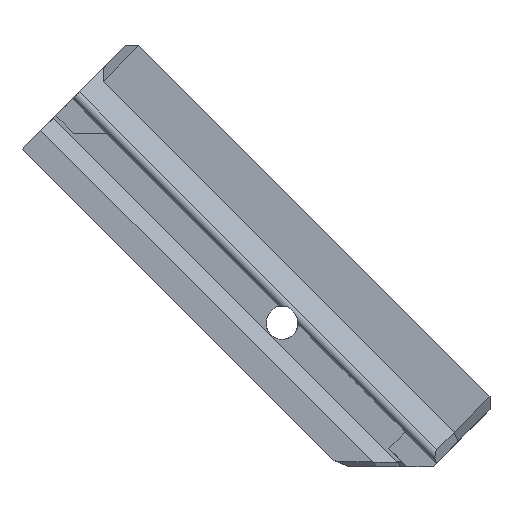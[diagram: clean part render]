
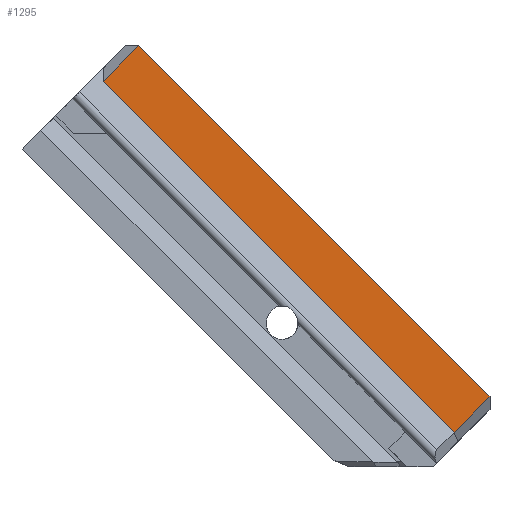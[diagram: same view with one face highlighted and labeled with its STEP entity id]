
A CAD part, left-side view. The second image highlights one B-rep face of the part: STEP entity #1295.
In plain terms, the highlighted planar face has unit normal (-1, 0, 0).
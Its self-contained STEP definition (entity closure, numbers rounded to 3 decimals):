
#69=FACE_OUTER_BOUND('',#141,.T.);
#141=EDGE_LOOP('',(#921,#922,#923,#924));
#245=LINE('',#1895,#410);
#255=LINE('',#1916,#420);
#259=LINE('',#1924,#424);
#260=LINE('',#1925,#425);
#410=VECTOR('',#1521,10.);
#420=VECTOR('',#1543,10.);
#424=VECTOR('',#1549,10.);
#425=VECTOR('',#1550,10.);
#567=VERTEX_POINT('',#1884);
#568=VERTEX_POINT('',#1889);
#574=VERTEX_POINT('',#1915);
#577=VERTEX_POINT('',#1923);
#695=EDGE_CURVE('',#567,#568,#245,.T.);
#705=EDGE_CURVE('',#568,#574,#255,.T.);
#709=EDGE_CURVE('',#567,#577,#259,.T.);
#710=EDGE_CURVE('',#574,#577,#260,.T.);
#921=ORIENTED_EDGE('',*,*,#695,.F.);
#922=ORIENTED_EDGE('',*,*,#709,.T.);
#923=ORIENTED_EDGE('',*,*,#710,.F.);
#924=ORIENTED_EDGE('',*,*,#705,.F.);
#1231=PLANE('',#1383);
#1295=ADVANCED_FACE('',(#69),#1231,.F.);
#1383=AXIS2_PLACEMENT_3D('',#1922,#1547,#1548);
#1521=DIRECTION('',(0.,0.707,-0.707));
#1543=DIRECTION('',(0.,0.707,0.707));
#1547=DIRECTION('center_axis',(1.,0.,0.));
#1548=DIRECTION('ref_axis',(0.,0.707,0.707));
#1549=DIRECTION('',(0.,0.707,0.707));
#1550=DIRECTION('',(0.,-0.707,0.707));
#1884=CARTESIAN_POINT('',(-8.23,12.159,9.993));
#1889=CARTESIAN_POINT('',(-8.23,15.971,6.181));
#1895=CARTESIAN_POINT('',(-8.23,11.207,10.945));
#1915=CARTESIAN_POINT('',(-8.23,53.235,43.446));
#1916=CARTESIAN_POINT('',(-8.23,46.871,37.082));
#1922=CARTESIAN_POINT('Origin',(-8.23,36.14,28.579));
#1923=CARTESIAN_POINT('',(-8.23,49.423,47.257));
#1924=CARTESIAN_POINT('',(-8.23,43.06,40.893));
#1925=CARTESIAN_POINT('',(-8.23,53.698,42.983));
